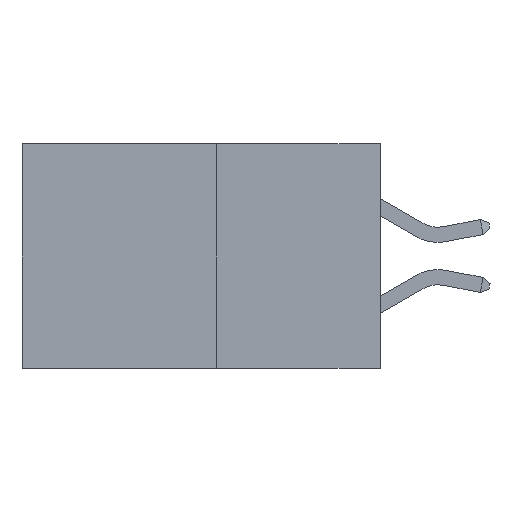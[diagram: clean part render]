
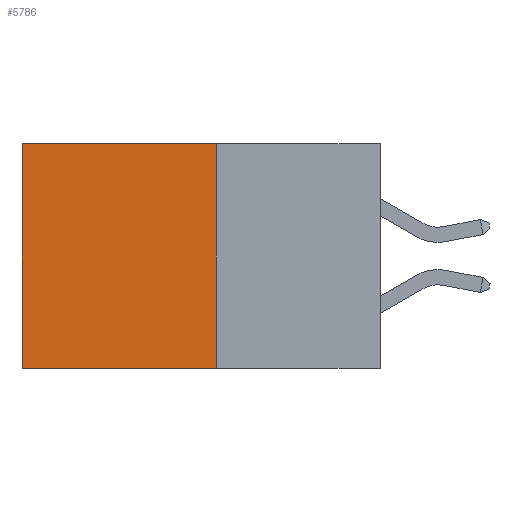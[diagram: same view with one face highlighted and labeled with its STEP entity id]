
A CAD part, left-side view. The second image highlights one B-rep face of the part: STEP entity #5786.
In plain terms, the highlighted planar face has unit normal (-1, 0, 0).
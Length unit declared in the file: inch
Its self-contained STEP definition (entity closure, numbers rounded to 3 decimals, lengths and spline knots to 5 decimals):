
#424 = AXIS2_PLACEMENT_3D ( 'NONE', #9208, #9027, #8936 ) ;
#2105 = EDGE_CURVE ( 'NONE', #19949, #5778, #15176, .T. ) ;
#3145 = CARTESIAN_POINT ( 'NONE',  ( 0.277, 0.27, -0.37 ) ) ;
#3446 = LINE ( 'NONE', #9583, #8376 ) ;
#3946 = VECTOR ( 'NONE', #9316, 39.37008 ) ;
#5561 = VECTOR ( 'NONE', #21534, 39.37008 ) ;
#5759 = EDGE_CURVE ( 'NONE', #15719, #19949, #3446, .T. ) ;
#5778 = VERTEX_POINT ( 'NONE', #9681 ) ;
#5786 = ADVANCED_FACE ( 'NONE', ( #25114 ), #9061, .F. ) ;
#7556 = VECTOR ( 'NONE', #12557, 39.37008 ) ;
#8376 = VECTOR ( 'NONE', #9529, 39.37008 ) ;
#8594 = EDGE_CURVE ( 'NONE', #20993, #5778, #12560, .T. ) ;
#8936 = DIRECTION ( 'NONE',  ( 0., 0., -1. ) ) ;
#9027 = DIRECTION ( 'NONE',  ( 1., 0., 0. ) ) ;
#9036 = ORIENTED_EDGE ( 'NONE', *, *, #9369, .F. ) ;
#9061 = PLANE ( 'NONE',  #424 ) ;
#9208 = CARTESIAN_POINT ( 'NONE',  ( 0.277, 0.27, -0.37 ) ) ;
#9316 = DIRECTION ( 'NONE',  ( 0., 0., -1. ) ) ;
#9369 = EDGE_CURVE ( 'NONE', #15719, #20993, #12568, .T. ) ;
#9529 = DIRECTION ( 'NONE',  ( 0., 1., 0. ) ) ;
#9583 = CARTESIAN_POINT ( 'NONE',  ( 0.277, 0.27, 0. ) ) ;
#9681 = CARTESIAN_POINT ( 'NONE',  ( 0.277, 0.59, -0.37 ) ) ;
#9696 = ORIENTED_EDGE ( 'NONE', *, *, #2105, .T. ) ;
#10452 = CARTESIAN_POINT ( 'NONE',  ( 0.277, 0.59, 0. ) ) ;
#10887 = ORIENTED_EDGE ( 'NONE', *, *, #8594, .F. ) ;
#12557 = DIRECTION ( 'NONE',  ( 0., 1., 0. ) ) ;
#12560 = LINE ( 'NONE', #27034, #7556 ) ;
#12568 = LINE ( 'NONE', #17382, #5561 ) ;
#15176 = LINE ( 'NONE', #23865, #3946 ) ;
#15719 = VERTEX_POINT ( 'NONE', #21913 ) ;
#17382 = CARTESIAN_POINT ( 'NONE',  ( 0.277, 0.27, -0.37 ) ) ;
#19047 = ORIENTED_EDGE ( 'NONE', *, *, #5759, .T. ) ;
#19949 = VERTEX_POINT ( 'NONE', #10452 ) ;
#20993 = VERTEX_POINT ( 'NONE', #3145 ) ;
#21534 = DIRECTION ( 'NONE',  ( 0., 0., -1. ) ) ;
#21913 = CARTESIAN_POINT ( 'NONE',  ( 0.277, 0.27, 0. ) ) ;
#22319 = EDGE_LOOP ( 'NONE', ( #9696, #10887, #9036, #19047 ) ) ;
#23865 = CARTESIAN_POINT ( 'NONE',  ( 0.277, 0.59, -0.37 ) ) ;
#25114 = FACE_OUTER_BOUND ( 'NONE', #22319, .T. ) ;
#27034 = CARTESIAN_POINT ( 'NONE',  ( 0.277, 0.27, -0.37 ) ) ;
